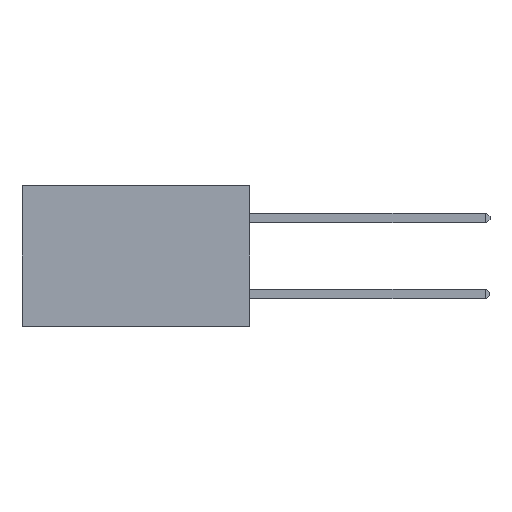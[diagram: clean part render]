
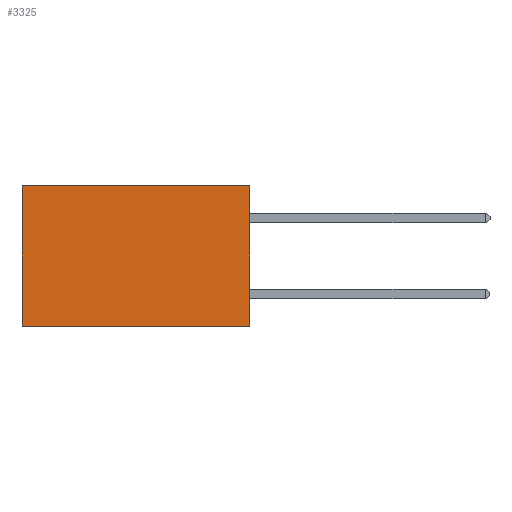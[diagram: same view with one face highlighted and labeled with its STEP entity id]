
A CAD part, left-side view. The second image highlights one B-rep face of the part: STEP entity #3325.
In plain terms, the highlighted planar face has unit normal (-1, 0, 0).
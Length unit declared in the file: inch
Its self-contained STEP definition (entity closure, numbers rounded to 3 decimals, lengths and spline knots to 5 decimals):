
#10 = VECTOR ( 'NONE', #2571, 39.37008 ) ;
#573 = AXIS2_PLACEMENT_3D ( 'NONE', #12168, #15166, #6169 ) ;
#1546 = CARTESIAN_POINT ( 'NONE',  ( 0.2875, 0.6, -0.37 ) ) ;
#1608 = ORIENTED_EDGE ( 'NONE', *, *, #6176, .F. ) ;
#2571 = DIRECTION ( 'NONE',  ( 0., 1., 0. ) ) ;
#3128 = VECTOR ( 'NONE', #5717, 39.37008 ) ;
#3325 = ADVANCED_FACE ( 'NONE', ( #14721 ), #15111, .F. ) ;
#3419 = EDGE_LOOP ( 'NONE', ( #8075, #1608, #12248, #5076 ) ) ;
#3488 = VERTEX_POINT ( 'NONE', #18509 ) ;
#4374 = EDGE_CURVE ( 'NONE', #8206, #10441, #12820, .T. ) ;
#5076 = ORIENTED_EDGE ( 'NONE', *, *, #4374, .T. ) ;
#5297 = CARTESIAN_POINT ( 'NONE',  ( 0.2875, 0., 0. ) ) ;
#5717 = DIRECTION ( 'NONE',  ( 0., 0., -1. ) ) ;
#6141 = DIRECTION ( 'NONE',  ( 0., 1., 0. ) ) ;
#6169 = DIRECTION ( 'NONE',  ( 0., 0., -1. ) ) ;
#6176 = EDGE_CURVE ( 'NONE', #3488, #9402, #16253, .T. ) ;
#7408 = CARTESIAN_POINT ( 'NONE',  ( 0.2875, 0.6, 0. ) ) ;
#7791 = CARTESIAN_POINT ( 'NONE',  ( 0.2875, 0., 0. ) ) ;
#8075 = ORIENTED_EDGE ( 'NONE', *, *, #10377, .T. ) ;
#8206 = VERTEX_POINT ( 'NONE', #7791 ) ;
#8350 = DIRECTION ( 'NONE',  ( 0., 0., -1. ) ) ;
#8823 = CARTESIAN_POINT ( 'NONE',  ( 0.2875, 0.6, 0. ) ) ;
#9402 = VERTEX_POINT ( 'NONE', #1546 ) ;
#10377 = EDGE_CURVE ( 'NONE', #10441, #9402, #10780, .T. ) ;
#10441 = VERTEX_POINT ( 'NONE', #7408 ) ;
#10780 = LINE ( 'NONE', #8823, #3128 ) ;
#11393 = LINE ( 'NONE', #5297, #14859 ) ;
#12168 = CARTESIAN_POINT ( 'NONE',  ( 0.2875, 0., 0. ) ) ;
#12248 = ORIENTED_EDGE ( 'NONE', *, *, #12613, .F. ) ;
#12613 = EDGE_CURVE ( 'NONE', #8206, #3488, #11393, .T. ) ;
#12820 = LINE ( 'NONE', #13807, #16318 ) ;
#13807 = CARTESIAN_POINT ( 'NONE',  ( 0.2875, 0., 0. ) ) ;
#14721 = FACE_OUTER_BOUND ( 'NONE', #3419, .T. ) ;
#14859 = VECTOR ( 'NONE', #8350, 39.37008 ) ;
#15111 = PLANE ( 'NONE',  #573 ) ;
#15166 = DIRECTION ( 'NONE',  ( 1., 0., 0. ) ) ;
#16253 = LINE ( 'NONE', #19225, #10 ) ;
#16318 = VECTOR ( 'NONE', #6141, 39.37008 ) ;
#18509 = CARTESIAN_POINT ( 'NONE',  ( 0.2875, 0., -0.37 ) ) ;
#19225 = CARTESIAN_POINT ( 'NONE',  ( 0.2875, 0., -0.37 ) ) ;
